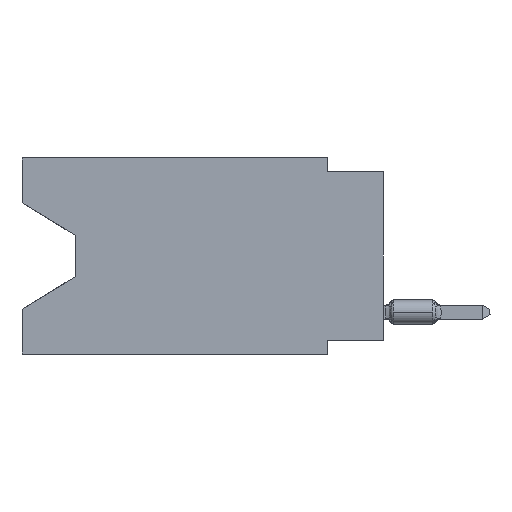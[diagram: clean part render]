
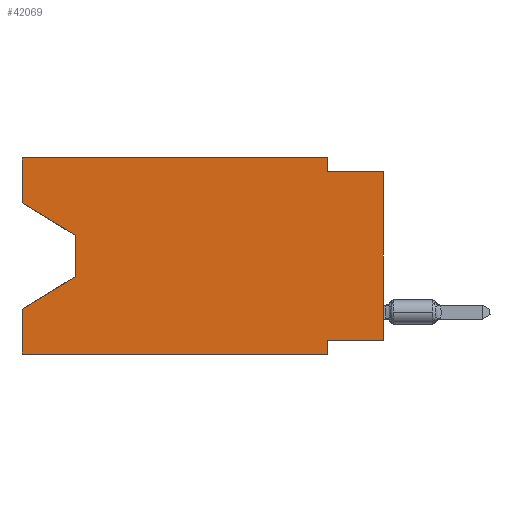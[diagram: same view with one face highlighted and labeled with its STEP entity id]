
A CAD part, left-side view. The second image highlights one B-rep face of the part: STEP entity #42069.
In plain terms, the highlighted planar face has unit normal (-1, 0, 0).
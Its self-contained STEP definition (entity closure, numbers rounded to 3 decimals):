
#1689 = EDGE_CURVE ( 'NONE', #31478, #49421, #11933, .T. ) ;
#2378 = VERTEX_POINT ( 'NONE', #5171 ) ;
#2460 = CARTESIAN_POINT ( 'NONE',  ( 0., 16.383, 0. ) ) ;
#3451 = VECTOR ( 'NONE', #58490, 1000. ) ;
#5103 = VECTOR ( 'NONE', #26697, 1000. ) ;
#5171 = CARTESIAN_POINT ( 'NONE',  ( 0., 0., -8.255 ) ) ;
#5217 = CARTESIAN_POINT ( 'NONE',  ( 0., 16.383, -2.038 ) ) ;
#5764 = EDGE_CURVE ( 'NONE', #52650, #27247, #60488, .T. ) ;
#7127 = LINE ( 'NONE', #17439, #36490 ) ;
#9633 = CARTESIAN_POINT ( 'NONE',  ( 0., 13.97, -5.385 ) ) ;
#9942 = CARTESIAN_POINT ( 'NONE',  ( 0., 16.383, 0. ) ) ;
#10805 = DIRECTION ( 'NONE',  ( 0., 0., -1. ) ) ;
#11377 = CARTESIAN_POINT ( 'NONE',  ( 0., 0., -8.255 ) ) ;
#11933 = LINE ( 'NONE', #32506, #5103 ) ;
#12773 = VERTEX_POINT ( 'NONE', #9942 ) ;
#13292 = CARTESIAN_POINT ( 'NONE',  ( 0., 13.97, -5.385 ) ) ;
#14032 = VECTOR ( 'NONE', #44129, 1000. ) ;
#15072 = EDGE_CURVE ( 'NONE', #12773, #31478, #59187, .T. ) ;
#15458 = LINE ( 'NONE', #20954, #35242 ) ;
#16093 = CARTESIAN_POINT ( 'NONE',  ( 0., 16.383, -2.038 ) ) ;
#16203 = DIRECTION ( 'NONE',  ( 0., 1., 0. ) ) ;
#16252 = VECTOR ( 'NONE', #33012, 1000. ) ;
#16619 = DIRECTION ( 'NONE',  ( 0., -1., 0. ) ) ;
#17400 = EDGE_LOOP ( 'NONE', ( #60068, #40145, #39143, #26113, #28420, #35347, #55527, #23957, #53054, #34935, #20297, #51208 ) ) ;
#17439 = CARTESIAN_POINT ( 'NONE',  ( 0., 16.383, 0. ) ) ;
#18110 = DIRECTION ( 'NONE',  ( 0., 0.855, -0.519 ) ) ;
#18613 = DIRECTION ( 'NONE',  ( 0., -1., 0. ) ) ;
#18960 = VERTEX_POINT ( 'NONE', #24560 ) ;
#20107 = EDGE_CURVE ( 'NONE', #67226, #27247, #53752, .T. ) ;
#20297 = ORIENTED_EDGE ( 'NONE', *, *, #15072, .F. ) ;
#20685 = LINE ( 'NONE', #11377, #29955 ) ;
#20954 = CARTESIAN_POINT ( 'NONE',  ( 0., 13.97, -3.505 ) ) ;
#22195 = CARTESIAN_POINT ( 'NONE',  ( 0., 2.54, -8.89 ) ) ;
#23753 = CARTESIAN_POINT ( 'NONE',  ( 0., 2.54, -8.255 ) ) ;
#23957 = ORIENTED_EDGE ( 'NONE', *, *, #52340, .T. ) ;
#24560 = CARTESIAN_POINT ( 'NONE',  ( 0., 13.97, -3.505 ) ) ;
#26113 = ORIENTED_EDGE ( 'NONE', *, *, #30238, .F. ) ;
#26697 = DIRECTION ( 'NONE',  ( 0., 0., -1. ) ) ;
#27247 = VERTEX_POINT ( 'NONE', #64515 ) ;
#27291 = DIRECTION ( 'NONE',  ( 1., 0., 0. ) ) ;
#27592 = LINE ( 'NONE', #48537, #3451 ) ;
#28420 = ORIENTED_EDGE ( 'NONE', *, *, #5764, .T. ) ;
#28537 = CARTESIAN_POINT ( 'NONE',  ( 0., 0., -0.635 ) ) ;
#29246 = CARTESIAN_POINT ( 'NONE',  ( 0., 16.383, -8.89 ) ) ;
#29955 = VECTOR ( 'NONE', #16203, 1000. ) ;
#30238 = EDGE_CURVE ( 'NONE', #52650, #65125, #48825, .T. ) ;
#31478 = VERTEX_POINT ( 'NONE', #64338 ) ;
#31704 = EDGE_CURVE ( 'NONE', #2378, #67226, #20685, .T. ) ;
#32314 = DIRECTION ( 'NONE',  ( 0., -0.855, -0.519 ) ) ;
#32347 = VERTEX_POINT ( 'NONE', #28537 ) ;
#32506 = CARTESIAN_POINT ( 'NONE',  ( 0., 2.54, 0. ) ) ;
#32805 = VECTOR ( 'NONE', #16619, 1000. ) ;
#33012 = DIRECTION ( 'NONE',  ( 0., 0., 1. ) ) ;
#33068 = CARTESIAN_POINT ( 'NONE',  ( 0., 16.383, 0. ) ) ;
#33459 = CARTESIAN_POINT ( 'NONE',  ( 0., 0., 0. ) ) ;
#34205 = VECTOR ( 'NONE', #18613, 1000. ) ;
#34935 = ORIENTED_EDGE ( 'NONE', *, *, #1689, .F. ) ;
#35242 = VECTOR ( 'NONE', #41870, 1000. ) ;
#35347 = ORIENTED_EDGE ( 'NONE', *, *, #20107, .F. ) ;
#36490 = VECTOR ( 'NONE', #58976, 1000. ) ;
#36967 = VECTOR ( 'NONE', #18110, 1000. ) ;
#37361 = VERTEX_POINT ( 'NONE', #9633 ) ;
#38955 = LINE ( 'NONE', #33459, #67844 ) ;
#39143 = ORIENTED_EDGE ( 'NONE', *, *, #51975, .T. ) ;
#40145 = ORIENTED_EDGE ( 'NONE', *, *, #57119, .T. ) ;
#40613 = CARTESIAN_POINT ( 'NONE',  ( 0., 16.383, -6.852 ) ) ;
#41460 = VECTOR ( 'NONE', #32314, 1000. ) ;
#41870 = DIRECTION ( 'NONE',  ( 0., 0., -1. ) ) ;
#42069 = ADVANCED_FACE ( 'NONE', ( #48564 ), #48234, .F. ) ;
#42379 = CARTESIAN_POINT ( 'NONE',  ( 0., 16.383, 0. ) ) ;
#44129 = DIRECTION ( 'NONE',  ( 0., 0., -1. ) ) ;
#47485 = CARTESIAN_POINT ( 'NONE',  ( 0., 16.383, -8.89 ) ) ;
#48234 = PLANE ( 'NONE',  #63643 ) ;
#48537 = CARTESIAN_POINT ( 'NONE',  ( 0., 0., -0.635 ) ) ;
#48564 = FACE_OUTER_BOUND ( 'NONE', #17400, .T. ) ;
#48825 = LINE ( 'NONE', #2460, #16252 ) ;
#49421 = VERTEX_POINT ( 'NONE', #51170 ) ;
#51170 = CARTESIAN_POINT ( 'NONE',  ( 0., 2.54, -0.635 ) ) ;
#51208 = ORIENTED_EDGE ( 'NONE', *, *, #58835, .F. ) ;
#51975 = EDGE_CURVE ( 'NONE', #37361, #65125, #55521, .T. ) ;
#52340 = EDGE_CURVE ( 'NONE', #2378, #32347, #38955, .T. ) ;
#52650 = VERTEX_POINT ( 'NONE', #47485 ) ;
#53054 = ORIENTED_EDGE ( 'NONE', *, *, #55092, .F. ) ;
#53752 = LINE ( 'NONE', #22195, #14032 ) ;
#54675 = VERTEX_POINT ( 'NONE', #16093 ) ;
#55092 = EDGE_CURVE ( 'NONE', #49421, #32347, #27592, .T. ) ;
#55521 = LINE ( 'NONE', #13292, #36967 ) ;
#55527 = ORIENTED_EDGE ( 'NONE', *, *, #31704, .F. ) ;
#57119 = EDGE_CURVE ( 'NONE', #18960, #37361, #15458, .T. ) ;
#58490 = DIRECTION ( 'NONE',  ( 0., -1., 0. ) ) ;
#58835 = EDGE_CURVE ( 'NONE', #54675, #12773, #7127, .T. ) ;
#58976 = DIRECTION ( 'NONE',  ( 0., 0., 1. ) ) ;
#59187 = LINE ( 'NONE', #33068, #32805 ) ;
#60068 = ORIENTED_EDGE ( 'NONE', *, *, #65215, .T. ) ;
#60488 = LINE ( 'NONE', #29246, #34205 ) ;
#63643 = AXIS2_PLACEMENT_3D ( 'NONE', #42379, #27291, #10805 ) ;
#64338 = CARTESIAN_POINT ( 'NONE',  ( 0., 2.54, 0. ) ) ;
#64515 = CARTESIAN_POINT ( 'NONE',  ( 0., 2.54, -8.89 ) ) ;
#65125 = VERTEX_POINT ( 'NONE', #40613 ) ;
#65215 = EDGE_CURVE ( 'NONE', #54675, #18960, #67713, .T. ) ;
#65741 = DIRECTION ( 'NONE',  ( 0., 0., 1. ) ) ;
#67226 = VERTEX_POINT ( 'NONE', #23753 ) ;
#67713 = LINE ( 'NONE', #5217, #41460 ) ;
#67844 = VECTOR ( 'NONE', #65741, 1000. ) ;
